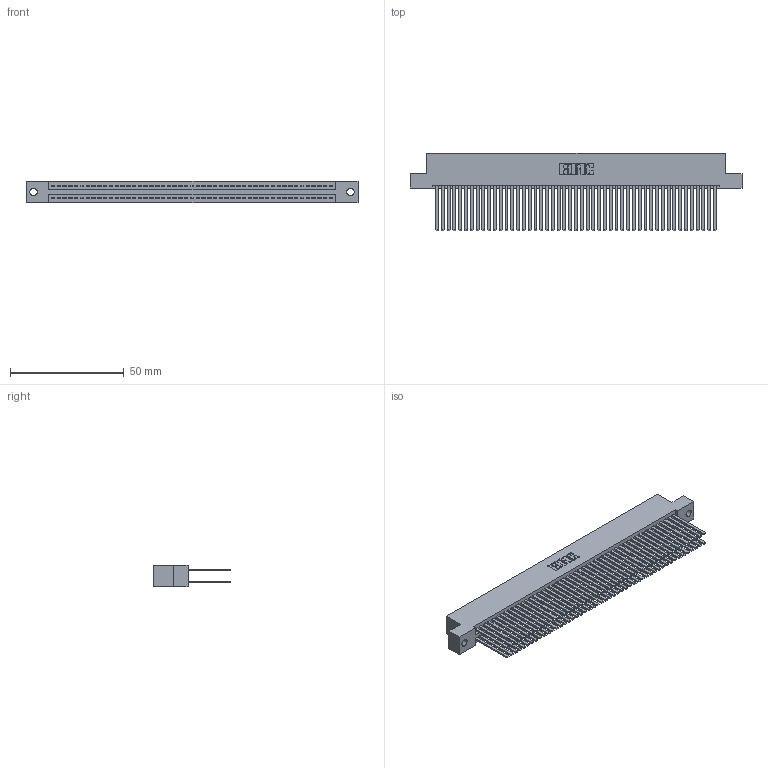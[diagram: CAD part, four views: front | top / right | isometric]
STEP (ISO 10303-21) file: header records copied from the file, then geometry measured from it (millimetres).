
FILE_DESCRIPTION (( 'STEP AP203' ), '1' );
FILE_NAME ('395-098-544-202.STEP', '2019-10-26T13:29:26', ( '' ), ( '' ), 'SwSTEP 2.0', 'SolidWorks 2016', '' );
FILE_SCHEMA (( 'CONFIG_CONTROL_DESIGN' ));
Length unit declared in the file: inch
Products named in the file (3): 345 Part_Flush Mounting Lugs - 0.128 Dia; 345-292-001_345-293-144; 395-098-544-202
Assembly tree (99 placements, depth 2):
  395-098-544-202
    345 Part_Flush Mounting Lugs - 0.128 Dia
    345-292-001_345-293-144  x98
Bounding box: 145.67 x 33.96 x 9.4 mm (x, y, z)
Volume: 15552.5 mm3; surface area: 26878.5 mm2
Topology: 99 solids, 99 shells, 4438 faces, 13179 edges, 8654 vertices
Faces by surface type: plane 2922, cylinder 1516
Entity records: 37323 total; most frequent: CARTESIAN_POINT 6248, ORIENTED_EDGE 6182, DIRECTION 5499, EDGE_CURVE 3091, VECTOR 2767, LINE 2767, VERTEX_POINT 2058, AXIS2_PLACEMENT_3D 1366
